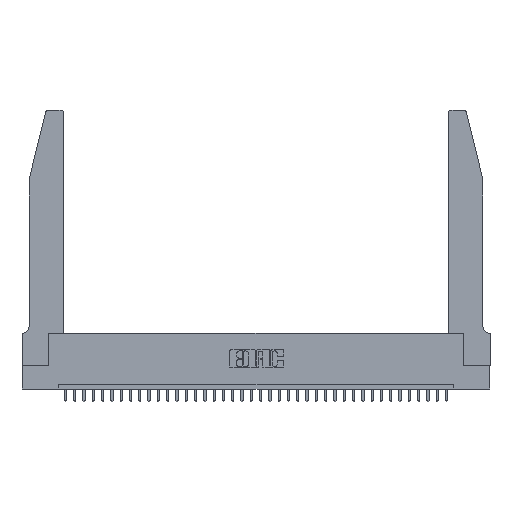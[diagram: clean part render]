
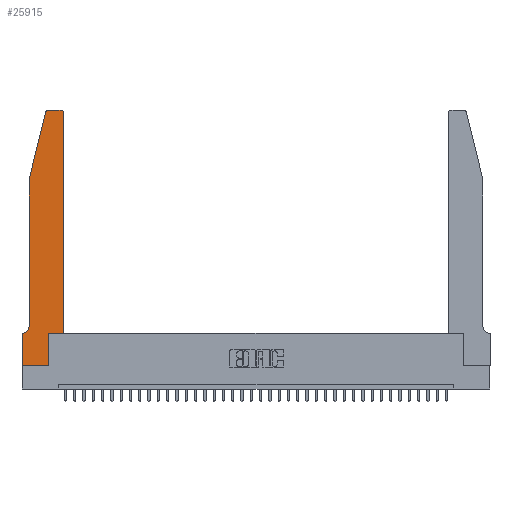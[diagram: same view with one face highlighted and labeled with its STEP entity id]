
A CAD part, top view. The second image highlights one B-rep face of the part: STEP entity #25915.
In plain terms, the highlighted planar face has unit normal (0, 0, 1).
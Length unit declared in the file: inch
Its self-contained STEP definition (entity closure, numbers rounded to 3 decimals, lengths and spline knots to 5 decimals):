
#83 = CIRCLE ( 'NONE', #25984, 0.03 ) ;
#310 = VECTOR ( 'NONE', #28087, 39.37008 ) ;
#1444 = CARTESIAN_POINT ( 'NONE',  ( 0.2865, 0.35, 0.37 ) ) ;
#1544 = VECTOR ( 'NONE', #7295, 39.37008 ) ;
#2164 = DIRECTION ( 'NONE',  ( -1., 0., 0. ) ) ;
#2531 = CARTESIAN_POINT ( 'NONE',  ( 0., 0.35, 0.37 ) ) ;
#2740 = CARTESIAN_POINT ( 'NONE',  ( 0.4505, 0.35, 0.37 ) ) ;
#2983 = EDGE_CURVE ( 'NONE', #4271, #7035, #17893, .T. ) ;
#3146 = CARTESIAN_POINT ( 'NONE',  ( 0.4505, 0.35, 0.37 ) ) ;
#3557 = ORIENTED_EDGE ( 'NONE', *, *, #34342, .T. ) ;
#3669 = LINE ( 'NONE', #5227, #25161 ) ;
#4271 = VERTEX_POINT ( 'NONE', #1444 ) ;
#4517 = CARTESIAN_POINT ( 'NONE',  ( 0.284, 2.72, 0.37 ) ) ;
#5227 = CARTESIAN_POINT ( 'NONE',  ( 0.0755, 2., 0.37 ) ) ;
#7035 = VERTEX_POINT ( 'NONE', #2740 ) ;
#7182 = DIRECTION ( 'NONE',  ( 0., 0., -1. ) ) ;
#7271 = DIRECTION ( 'NONE',  ( 0., 0., 1. ) ) ;
#7295 = DIRECTION ( 'NONE',  ( 0., -1., 0. ) ) ;
#7325 = CARTESIAN_POINT ( 'NONE',  ( 0.2865, 0., 0.37 ) ) ;
#7546 = DIRECTION ( 'NONE',  ( 0., -1., 0. ) ) ;
#7722 = CARTESIAN_POINT ( 'NONE',  ( 0.4505, 0.35, 0.37 ) ) ;
#7875 = VECTOR ( 'NONE', #11290, 39.37008 ) ;
#8088 = EDGE_CURVE ( 'NONE', #36260, #22785, #28763, .T. ) ;
#9143 = EDGE_CURVE ( 'NONE', #15153, #9478, #83, .T. ) ;
#9478 = VERTEX_POINT ( 'NONE', #14682 ) ;
#9892 = LINE ( 'NONE', #10452, #24844 ) ;
#9919 = CIRCLE ( 'NONE', #25884, 0.03 ) ;
#10452 = CARTESIAN_POINT ( 'NONE',  ( 0.2605, 2.75, 0.37 ) ) ;
#11056 = ORIENTED_EDGE ( 'NONE', *, *, #32749, .T. ) ;
#11290 = DIRECTION ( 'NONE',  ( 1., 0., 0. ) ) ;
#12692 = ORIENTED_EDGE ( 'NONE', *, *, #9143, .T. ) ;
#12888 = CARTESIAN_POINT ( 'NONE',  ( 0.4205, 2.72, 0.37 ) ) ;
#13177 = CARTESIAN_POINT ( 'NONE',  ( 0.0755, 0.35, 0.37 ) ) ;
#14682 = CARTESIAN_POINT ( 'NONE',  ( 0.4205, 2.75, 0.37 ) ) ;
#14709 = CARTESIAN_POINT ( 'NONE',  ( 0.0055, 0.35, 0.37 ) ) ;
#14796 = CIRCLE ( 'NONE', #32381, 0.07 ) ;
#14974 = EDGE_CURVE ( 'NONE', #7035, #15153, #26858, .T. ) ;
#15138 = CARTESIAN_POINT ( 'NONE',  ( 0.0055, 0.42, 0.37 ) ) ;
#15153 = VERTEX_POINT ( 'NONE', #30566 ) ;
#15226 = EDGE_CURVE ( 'NONE', #34277, #4271, #15393, .T. ) ;
#15393 = LINE ( 'NONE', #23067, #17161 ) ;
#15793 = CARTESIAN_POINT ( 'NONE',  ( 0.0755, 0.42, 0.37 ) ) ;
#15981 = CARTESIAN_POINT ( 'NONE',  ( 0., 0., 0.37 ) ) ;
#16274 = ORIENTED_EDGE ( 'NONE', *, *, #34012, .T. ) ;
#16413 = DIRECTION ( 'NONE',  ( -0.239, -0.971, 0. ) ) ;
#17161 = VECTOR ( 'NONE', #26753, 39.37008 ) ;
#17540 = EDGE_CURVE ( 'NONE', #33160, #30518, #9919, .T. ) ;
#17668 = VERTEX_POINT ( 'NONE', #15793 ) ;
#17893 = LINE ( 'NONE', #3146, #310 ) ;
#17964 = VECTOR ( 'NONE', #2164, 39.37008 ) ;
#17990 = DIRECTION ( 'NONE',  ( 1., 0., 0. ) ) ;
#18694 = CARTESIAN_POINT ( 'NONE',  ( 0.0755, 2., 0.37 ) ) ;
#18967 = CARTESIAN_POINT ( 'NONE',  ( 0.0755, 2., 0.37 ) ) ;
#19798 = VECTOR ( 'NONE', #32679, 39.37008 ) ;
#20008 = EDGE_CURVE ( 'NONE', #30518, #26370, #3669, .T. ) ;
#20156 = ORIENTED_EDGE ( 'NONE', *, *, #14974, .T. ) ;
#21456 = PLANE ( 'NONE',  #32428 ) ;
#21581 = CARTESIAN_POINT ( 'NONE',  ( 0., 0.35, 0.37 ) ) ;
#22403 = VERTEX_POINT ( 'NONE', #14709 ) ;
#22785 = VERTEX_POINT ( 'NONE', #33038 ) ;
#23067 = CARTESIAN_POINT ( 'NONE',  ( 0.2865, 0.35, 0.37 ) ) ;
#23445 = ORIENTED_EDGE ( 'NONE', *, *, #34353, .T. ) ;
#24122 = DIRECTION ( 'NONE',  ( 0., 0., 1. ) ) ;
#24844 = VECTOR ( 'NONE', #32744, 39.37008 ) ;
#25161 = VECTOR ( 'NONE', #16413, 39.37008 ) ;
#25845 = LINE ( 'NONE', #28599, #7875 ) ;
#25884 = AXIS2_PLACEMENT_3D ( 'NONE', #4517, #24122, #17990 ) ;
#25915 = ADVANCED_FACE ( 'NONE', ( #33021 ), #21456, .T. ) ;
#25984 = AXIS2_PLACEMENT_3D ( 'NONE', #12888, #26632, #32056 ) ;
#26370 = VERTEX_POINT ( 'NONE', #18694 ) ;
#26420 = DIRECTION ( 'NONE',  ( -1., 0., 0. ) ) ;
#26632 = DIRECTION ( 'NONE',  ( 0., 0., 1. ) ) ;
#26753 = DIRECTION ( 'NONE',  ( 0., 1., 0. ) ) ;
#26858 = LINE ( 'NONE', #7722, #19798 ) ;
#27329 = EDGE_LOOP ( 'NONE', ( #3557, #32255, #32349, #23445, #16274, #30713, #33317, #11056, #34480, #28112, #20156, #12692 ) ) ;
#28087 = DIRECTION ( 'NONE',  ( 1., 0., 0. ) ) ;
#28112 = ORIENTED_EDGE ( 'NONE', *, *, #2983, .T. ) ;
#28366 = LINE ( 'NONE', #18967, #32787 ) ;
#28599 = CARTESIAN_POINT ( 'NONE',  ( 0., 0., 0.37 ) ) ;
#28763 = LINE ( 'NONE', #15981, #1544 ) ;
#30345 = CARTESIAN_POINT ( 'NONE',  ( 0.25487, 2.72718, 0.37 ) ) ;
#30518 = VERTEX_POINT ( 'NONE', #30345 ) ;
#30566 = CARTESIAN_POINT ( 'NONE',  ( 0.4505, 2.72, 0.37 ) ) ;
#30713 = ORIENTED_EDGE ( 'NONE', *, *, #32530, .T. ) ;
#32056 = DIRECTION ( 'NONE',  ( 1., 0., 0. ) ) ;
#32255 = ORIENTED_EDGE ( 'NONE', *, *, #17540, .T. ) ;
#32302 = DIRECTION ( 'NONE',  ( 1., 0., 0. ) ) ;
#32349 = ORIENTED_EDGE ( 'NONE', *, *, #20008, .T. ) ;
#32381 = AXIS2_PLACEMENT_3D ( 'NONE', #15138, #7182, #26420 ) ;
#32428 = AXIS2_PLACEMENT_3D ( 'NONE', #21581, #7271, #32302 ) ;
#32530 = EDGE_CURVE ( 'NONE', #22403, #36260, #35105, .T. ) ;
#32679 = DIRECTION ( 'NONE',  ( 0., 1., 0. ) ) ;
#32744 = DIRECTION ( 'NONE',  ( -1., 0., 0. ) ) ;
#32749 = EDGE_CURVE ( 'NONE', #22785, #34277, #25845, .T. ) ;
#32787 = VECTOR ( 'NONE', #7546, 39.37008 ) ;
#33021 = FACE_OUTER_BOUND ( 'NONE', #27329, .T. ) ;
#33038 = CARTESIAN_POINT ( 'NONE',  ( 0., 0., 0.37 ) ) ;
#33160 = VERTEX_POINT ( 'NONE', #33771 ) ;
#33317 = ORIENTED_EDGE ( 'NONE', *, *, #8088, .T. ) ;
#33771 = CARTESIAN_POINT ( 'NONE',  ( 0.284, 2.75, 0.37 ) ) ;
#34012 = EDGE_CURVE ( 'NONE', #17668, #22403, #14796, .T. ) ;
#34277 = VERTEX_POINT ( 'NONE', #7325 ) ;
#34342 = EDGE_CURVE ( 'NONE', #9478, #33160, #9892, .T. ) ;
#34353 = EDGE_CURVE ( 'NONE', #26370, #17668, #28366, .T. ) ;
#34480 = ORIENTED_EDGE ( 'NONE', *, *, #15226, .T. ) ;
#35105 = LINE ( 'NONE', #13177, #17964 ) ;
#36260 = VERTEX_POINT ( 'NONE', #2531 ) ;
